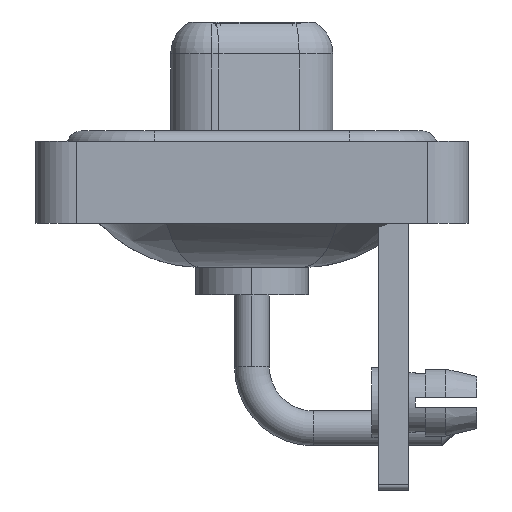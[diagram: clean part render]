
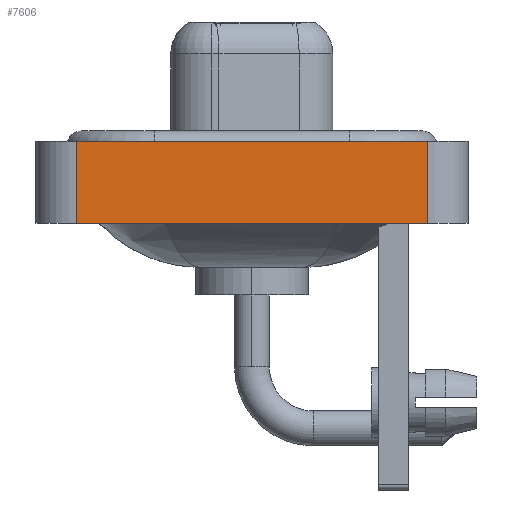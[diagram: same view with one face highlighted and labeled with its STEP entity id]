
A CAD part, left-side view. The second image highlights one B-rep face of the part: STEP entity #7606.
In plain terms, the highlighted planar face has unit normal (-1, 0, 0).
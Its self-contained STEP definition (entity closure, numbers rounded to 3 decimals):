
#156 = EDGE_CURVE ( 'NONE', #11796, #11668, #17062, .T. ) ;
#456 = DIRECTION ( 'NONE',  ( 0., -1., 0. ) ) ;
#992 = CARTESIAN_POINT ( 'NONE',  ( -7.3, -8.55, 0.4 ) ) ;
#1491 = CARTESIAN_POINT ( 'NONE',  ( -7.3, -8.55, 0.4 ) ) ;
#2211 = VERTEX_POINT ( 'NONE', #10742 ) ;
#2788 = CARTESIAN_POINT ( 'NONE',  ( -7.3, 8.55, 0.4 ) ) ;
#3188 = DIRECTION ( 'NONE',  ( 0., -1., 0. ) ) ;
#3375 = CARTESIAN_POINT ( 'NONE',  ( -7.3, 8.55, -3.6 ) ) ;
#4472 = VECTOR ( 'NONE', #3188, 1000. ) ;
#4604 = ORIENTED_EDGE ( 'NONE', *, *, #156, .F. ) ;
#4855 = VECTOR ( 'NONE', #456, 1000. ) ;
#5178 = LINE ( 'NONE', #11362, #4855 ) ;
#6022 = DIRECTION ( 'NONE',  ( 0., 0., 1. ) ) ;
#6133 = VECTOR ( 'NONE', #18446, 1000. ) ;
#6237 = EDGE_LOOP ( 'NONE', ( #10914, #4604, #9663, #8370 ) ) ;
#7606 = ADVANCED_FACE ( 'NONE', ( #16974 ), #13949, .T. ) ;
#8370 = ORIENTED_EDGE ( 'NONE', *, *, #10173, .T. ) ;
#8580 = EDGE_CURVE ( 'NONE', #17289, #11796, #11628, .T. ) ;
#8805 = VECTOR ( 'NONE', #17696, 1000. ) ;
#8916 = CARTESIAN_POINT ( 'NONE',  ( -7.3, -8.55, -3.6 ) ) ;
#9055 = DIRECTION ( 'NONE',  ( -1., 0., 0. ) ) ;
#9663 = ORIENTED_EDGE ( 'NONE', *, *, #8580, .F. ) ;
#9891 = CARTESIAN_POINT ( 'NONE',  ( -7.3, 8.55, -3.6 ) ) ;
#10173 = EDGE_CURVE ( 'NONE', #17289, #2211, #5178, .T. ) ;
#10559 = LINE ( 'NONE', #8916, #6133 ) ;
#10698 = CARTESIAN_POINT ( 'NONE',  ( -7.3, -8.55, -3.6 ) ) ;
#10742 = CARTESIAN_POINT ( 'NONE',  ( -7.3, -8.55, -3.6 ) ) ;
#10914 = ORIENTED_EDGE ( 'NONE', *, *, #13593, .T. ) ;
#11362 = CARTESIAN_POINT ( 'NONE',  ( -7.3, -8.55, -3.6 ) ) ;
#11628 = LINE ( 'NONE', #9891, #8805 ) ;
#11668 = VERTEX_POINT ( 'NONE', #992 ) ;
#11688 = AXIS2_PLACEMENT_3D ( 'NONE', #10698, #9055, #6022 ) ;
#11796 = VERTEX_POINT ( 'NONE', #2788 ) ;
#13593 = EDGE_CURVE ( 'NONE', #2211, #11668, #10559, .T. ) ;
#13949 = PLANE ( 'NONE',  #11688 ) ;
#16974 = FACE_OUTER_BOUND ( 'NONE', #6237, .T. ) ;
#17062 = LINE ( 'NONE', #1491, #4472 ) ;
#17289 = VERTEX_POINT ( 'NONE', #3375 ) ;
#17696 = DIRECTION ( 'NONE',  ( 0., 0., 1. ) ) ;
#18446 = DIRECTION ( 'NONE',  ( 0., 0., 1. ) ) ;
